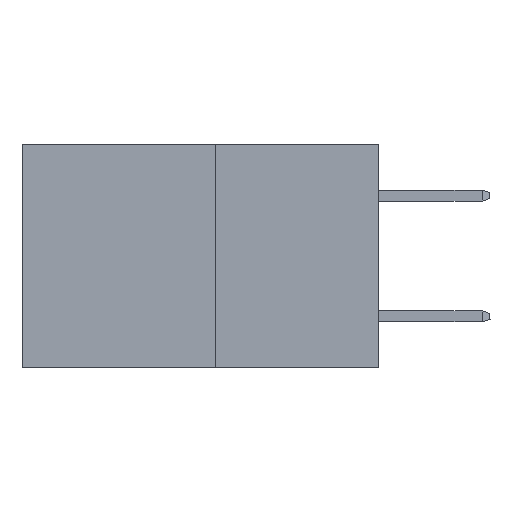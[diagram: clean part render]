
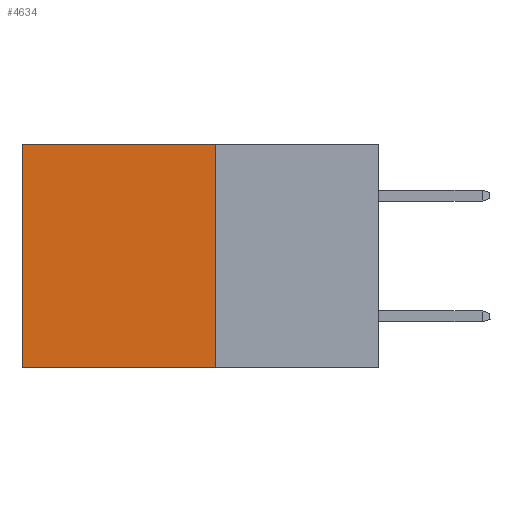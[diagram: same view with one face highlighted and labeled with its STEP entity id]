
A CAD part, left-side view. The second image highlights one B-rep face of the part: STEP entity #4634.
In plain terms, the highlighted planar face has unit normal (-1, 0, 0).
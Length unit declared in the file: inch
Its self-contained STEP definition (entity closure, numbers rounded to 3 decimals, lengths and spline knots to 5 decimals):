
#457 = LINE ( 'NONE', #18343, #20490 ) ;
#913 = DIRECTION ( 'NONE',  ( 0., 0., -1. ) ) ;
#1315 = CARTESIAN_POINT ( 'NONE',  ( 0.277, 0.27, -0.37 ) ) ;
#2204 = CARTESIAN_POINT ( 'NONE',  ( 0.277, 0.59, -0.37 ) ) ;
#2375 = VERTEX_POINT ( 'NONE', #1315 ) ;
#2641 = VECTOR ( 'NONE', #14424, 39.37008 ) ;
#3114 = CARTESIAN_POINT ( 'NONE',  ( 0.277, 0.27, -0.37 ) ) ;
#4167 = DIRECTION ( 'NONE',  ( 0., 0., -1. ) ) ;
#4634 = ADVANCED_FACE ( 'NONE', ( #21169 ), #24126, .F. ) ;
#4749 = DIRECTION ( 'NONE',  ( 0., 1., 0. ) ) ;
#5030 = LINE ( 'NONE', #3114, #14771 ) ;
#6005 = VERTEX_POINT ( 'NONE', #20299 ) ;
#6586 = VERTEX_POINT ( 'NONE', #16222 ) ;
#7214 = VECTOR ( 'NONE', #4167, 39.37008 ) ;
#7677 = AXIS2_PLACEMENT_3D ( 'NONE', #20250, #12539, #913 ) ;
#7776 = VERTEX_POINT ( 'NONE', #16089 ) ;
#10848 = ORIENTED_EDGE ( 'NONE', *, *, #11164, .F. ) ;
#11164 = EDGE_CURVE ( 'NONE', #2375, #7776, #12980, .T. ) ;
#11878 = ORIENTED_EDGE ( 'NONE', *, *, #21042, .T. ) ;
#12004 = EDGE_CURVE ( 'NONE', #6586, #2375, #5030, .T. ) ;
#12539 = DIRECTION ( 'NONE',  ( 1., 0., 0. ) ) ;
#12980 = LINE ( 'NONE', #20285, #2641 ) ;
#14424 = DIRECTION ( 'NONE',  ( 0., 1., 0. ) ) ;
#14751 = DIRECTION ( 'NONE',  ( 0., 0., -1. ) ) ;
#14771 = VECTOR ( 'NONE', #14751, 39.37008 ) ;
#15443 = ORIENTED_EDGE ( 'NONE', *, *, #12004, .F. ) ;
#16089 = CARTESIAN_POINT ( 'NONE',  ( 0.277, 0.59, -0.37 ) ) ;
#16222 = CARTESIAN_POINT ( 'NONE',  ( 0.277, 0.27, 0. ) ) ;
#16922 = EDGE_LOOP ( 'NONE', ( #11878, #10848, #15443, #23954 ) ) ;
#18343 = CARTESIAN_POINT ( 'NONE',  ( 0.277, 0.27, 0. ) ) ;
#20250 = CARTESIAN_POINT ( 'NONE',  ( 0.277, 0.27, -0.37 ) ) ;
#20285 = CARTESIAN_POINT ( 'NONE',  ( 0.277, 0.27, -0.37 ) ) ;
#20299 = CARTESIAN_POINT ( 'NONE',  ( 0.277, 0.59, 0. ) ) ;
#20490 = VECTOR ( 'NONE', #4749, 39.37008 ) ;
#21042 = EDGE_CURVE ( 'NONE', #6005, #7776, #22100, .T. ) ;
#21169 = FACE_OUTER_BOUND ( 'NONE', #16922, .T. ) ;
#22100 = LINE ( 'NONE', #2204, #7214 ) ;
#22614 = EDGE_CURVE ( 'NONE', #6586, #6005, #457, .T. ) ;
#23954 = ORIENTED_EDGE ( 'NONE', *, *, #22614, .T. ) ;
#24126 = PLANE ( 'NONE',  #7677 ) ;
